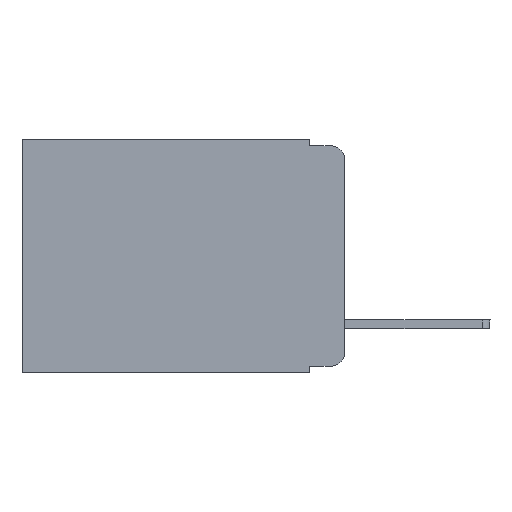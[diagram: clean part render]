
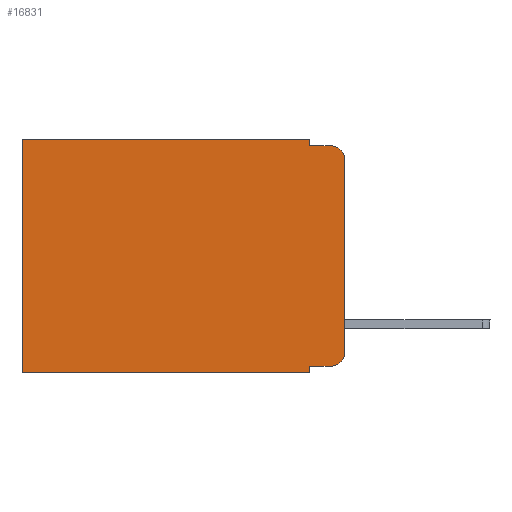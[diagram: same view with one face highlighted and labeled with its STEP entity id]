
A CAD part, left-side view. The second image highlights one B-rep face of the part: STEP entity #16831.
In plain terms, the highlighted planar face has unit normal (-1, 0, 0).
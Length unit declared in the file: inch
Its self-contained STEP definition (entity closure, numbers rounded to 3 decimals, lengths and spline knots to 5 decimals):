
#164 = CARTESIAN_POINT ( 'NONE',  ( 0.298, 0., -0.313 ) ) ;
#344 = EDGE_CURVE ( 'NONE', #14913, #7291, #15769, .T. ) ;
#458 = ORIENTED_EDGE ( 'NONE', *, *, #13112, .F. ) ;
#475 = CARTESIAN_POINT ( 'NONE',  ( 0.298, 0.051, 0. ) ) ;
#927 = AXIS2_PLACEMENT_3D ( 'NONE', #3817, #13922, #8310 ) ;
#983 = VECTOR ( 'NONE', #12140, 39.37008 ) ;
#1054 = DIRECTION ( 'NONE',  ( 0., -1., 0. ) ) ;
#1378 = EDGE_CURVE ( 'NONE', #13878, #1388, #15268, .T. ) ;
#1388 = VERTEX_POINT ( 'NONE', #2335 ) ;
#1431 = VECTOR ( 'NONE', #1054, 39.37008 ) ;
#2226 = ORIENTED_EDGE ( 'NONE', *, *, #16761, .F. ) ;
#2335 = CARTESIAN_POINT ( 'NONE',  ( 0.298, 0.02, -0.333 ) ) ;
#2483 = CARTESIAN_POINT ( 'NONE',  ( 0.298, 0.051, -0.333 ) ) ;
#2596 = VERTEX_POINT ( 'NONE', #16606 ) ;
#2808 = VECTOR ( 'NONE', #17766, 39.37008 ) ;
#2876 = CARTESIAN_POINT ( 'NONE',  ( 0.298, 0.473, 0. ) ) ;
#3344 = CARTESIAN_POINT ( 'NONE',  ( 0.298, 0., 0. ) ) ;
#3536 = ORIENTED_EDGE ( 'NONE', *, *, #1378, .T. ) ;
#3817 = CARTESIAN_POINT ( 'NONE',  ( 0.298, 0.02, -0.313 ) ) ;
#4252 = LINE ( 'NONE', #12882, #11255 ) ;
#4336 = DIRECTION ( 'NONE',  ( 0., 0., -1. ) ) ;
#4384 = LINE ( 'NONE', #7381, #2808 ) ;
#4398 = LINE ( 'NONE', #3344, #983 ) ;
#4426 = VECTOR ( 'NONE', #4336, 39.37008 ) ;
#4639 = ORIENTED_EDGE ( 'NONE', *, *, #344, .T. ) ;
#4759 = CARTESIAN_POINT ( 'NONE',  ( 0.298, 0., 0. ) ) ;
#5247 = VECTOR ( 'NONE', #9462, 39.37008 ) ;
#5411 = DIRECTION ( 'NONE',  ( 0., 0., -1. ) ) ;
#5435 = CARTESIAN_POINT ( 'NONE',  ( 0.298, 0.051, -0.333 ) ) ;
#5581 = FACE_OUTER_BOUND ( 'NONE', #7528, .T. ) ;
#5715 = CARTESIAN_POINT ( 'NONE',  ( 0.298, 0.051, -0.01 ) ) ;
#5978 = AXIS2_PLACEMENT_3D ( 'NONE', #4759, #10536, #9138 ) ;
#6151 = ORIENTED_EDGE ( 'NONE', *, *, #9989, .T. ) ;
#6813 = DIRECTION ( 'NONE',  ( 0., 0., -1. ) ) ;
#7213 = VERTEX_POINT ( 'NONE', #164 ) ;
#7291 = VERTEX_POINT ( 'NONE', #15110 ) ;
#7381 = CARTESIAN_POINT ( 'NONE',  ( 0.298, 0.051, 0. ) ) ;
#7528 = EDGE_LOOP ( 'NONE', ( #14991, #17578, #10088, #8041, #17468, #4639, #2226, #458, #3536, #6151 ) ) ;
#8041 = ORIENTED_EDGE ( 'NONE', *, *, #8451, .F. ) ;
#8310 = DIRECTION ( 'NONE',  ( 0., 0., -1. ) ) ;
#8312 = EDGE_CURVE ( 'NONE', #16297, #14913, #11825, .T. ) ;
#8324 = CARTESIAN_POINT ( 'NONE',  ( 0.298, 0., -0.03 ) ) ;
#8451 = EDGE_CURVE ( 'NONE', #16297, #18571, #18429, .T. ) ;
#8865 = VECTOR ( 'NONE', #5411, 39.37008 ) ;
#8935 = CARTESIAN_POINT ( 'NONE',  ( 0.298, 0.473, 0. ) ) ;
#9138 = DIRECTION ( 'NONE',  ( 0., 0., -1. ) ) ;
#9246 = CIRCLE ( 'NONE', #927, 0.02 ) ;
#9462 = DIRECTION ( 'NONE',  ( 0., 1., 0. ) ) ;
#9828 = EDGE_CURVE ( 'NONE', #18571, #2596, #13524, .T. ) ;
#9989 = EDGE_CURVE ( 'NONE', #1388, #7213, #9246, .T. ) ;
#10088 = ORIENTED_EDGE ( 'NONE', *, *, #9828, .F. ) ;
#10147 = VERTEX_POINT ( 'NONE', #11784 ) ;
#10343 = PLANE ( 'NONE',  #5978 ) ;
#10536 = DIRECTION ( 'NONE',  ( 1., 0., 0. ) ) ;
#11054 = DIRECTION ( 'NONE',  ( -1., 0., 0. ) ) ;
#11182 = CARTESIAN_POINT ( 'NONE',  ( 0.298, 0.051, 0. ) ) ;
#11255 = VECTOR ( 'NONE', #15939, 39.37008 ) ;
#11784 = CARTESIAN_POINT ( 'NONE',  ( 0.298, 0.051, -0.343 ) ) ;
#11805 = CIRCLE ( 'NONE', #17871, 0.02 ) ;
#11825 = LINE ( 'NONE', #12519, #5247 ) ;
#12140 = DIRECTION ( 'NONE',  ( 0., 0., -1. ) ) ;
#12519 = CARTESIAN_POINT ( 'NONE',  ( 0.298, 0., 0. ) ) ;
#12882 = CARTESIAN_POINT ( 'NONE',  ( 0.298, 0., -0.343 ) ) ;
#13112 = EDGE_CURVE ( 'NONE', #13878, #10147, #4384, .T. ) ;
#13467 = CARTESIAN_POINT ( 'NONE',  ( 0.298, 0.051, -0.01 ) ) ;
#13524 = LINE ( 'NONE', #13467, #18352 ) ;
#13878 = VERTEX_POINT ( 'NONE', #2483 ) ;
#13922 = DIRECTION ( 'NONE',  ( -1., 0., 0. ) ) ;
#14759 = EDGE_CURVE ( 'NONE', #17053, #2596, #11805, .T. ) ;
#14913 = VERTEX_POINT ( 'NONE', #8935 ) ;
#14968 = DIRECTION ( 'NONE',  ( 0., -1., 0. ) ) ;
#14991 = ORIENTED_EDGE ( 'NONE', *, *, #18215, .F. ) ;
#15110 = CARTESIAN_POINT ( 'NONE',  ( 0.298, 0.473, -0.343 ) ) ;
#15268 = LINE ( 'NONE', #5435, #1431 ) ;
#15769 = LINE ( 'NONE', #2876, #4426 ) ;
#15939 = DIRECTION ( 'NONE',  ( 0., 1., 0. ) ) ;
#16297 = VERTEX_POINT ( 'NONE', #475 ) ;
#16606 = CARTESIAN_POINT ( 'NONE',  ( 0.298, 0.02, -0.01 ) ) ;
#16761 = EDGE_CURVE ( 'NONE', #10147, #7291, #4252, .T. ) ;
#16831 = ADVANCED_FACE ( 'NONE', ( #5581 ), #10343, .F. ) ;
#17053 = VERTEX_POINT ( 'NONE', #8324 ) ;
#17468 = ORIENTED_EDGE ( 'NONE', *, *, #8312, .T. ) ;
#17578 = ORIENTED_EDGE ( 'NONE', *, *, #14759, .T. ) ;
#17766 = DIRECTION ( 'NONE',  ( 0., 0., -1. ) ) ;
#17871 = AXIS2_PLACEMENT_3D ( 'NONE', #18286, #11054, #6813 ) ;
#18215 = EDGE_CURVE ( 'NONE', #17053, #7213, #4398, .T. ) ;
#18286 = CARTESIAN_POINT ( 'NONE',  ( 0.298, 0.02, -0.03 ) ) ;
#18352 = VECTOR ( 'NONE', #14968, 39.37008 ) ;
#18429 = LINE ( 'NONE', #11182, #8865 ) ;
#18571 = VERTEX_POINT ( 'NONE', #5715 ) ;
